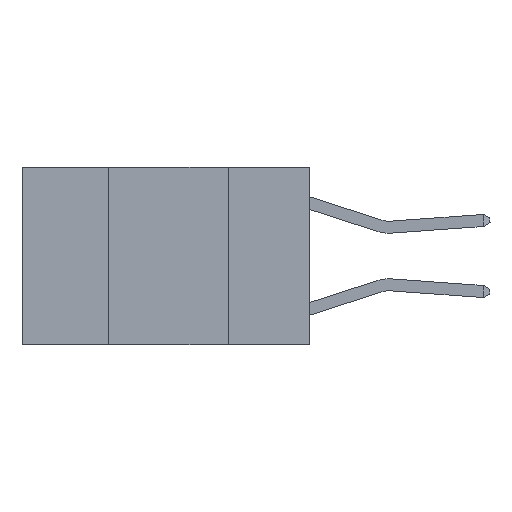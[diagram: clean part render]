
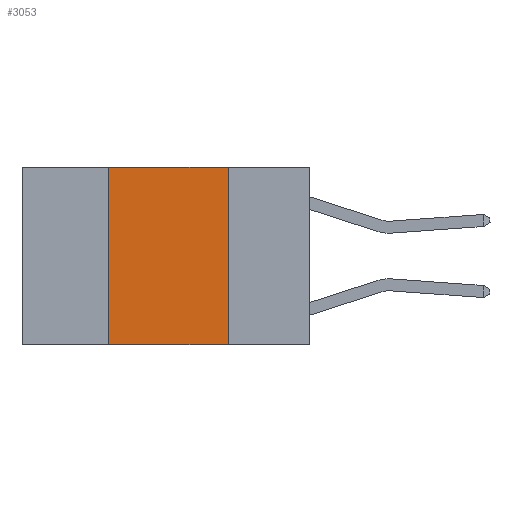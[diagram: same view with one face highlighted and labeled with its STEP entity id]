
A CAD part, left-side view. The second image highlights one B-rep face of the part: STEP entity #3053.
In plain terms, the highlighted planar face has unit normal (-1, 0, 0).
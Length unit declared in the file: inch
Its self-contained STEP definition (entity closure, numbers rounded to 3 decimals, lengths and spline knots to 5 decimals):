
#655 = VECTOR ( 'NONE', #10070, 39.37008 ) ;
#733 = PLANE ( 'NONE',  #889 ) ;
#889 = AXIS2_PLACEMENT_3D ( 'NONE', #7537, #8256, #3451 ) ;
#1529 = LINE ( 'NONE', #8002, #655 ) ;
#1813 = EDGE_CURVE ( 'NONE', #2491, #2219, #2151, .T. ) ;
#1826 = EDGE_LOOP ( 'NONE', ( #6441, #3651, #5259, #5713 ) ) ;
#2132 = CARTESIAN_POINT ( 'NONE',  ( 0., 0.6, 0. ) ) ;
#2151 = LINE ( 'NONE', #4082, #3375 ) ;
#2219 = VERTEX_POINT ( 'NONE', #6234 ) ;
#2269 = DIRECTION ( 'NONE',  ( 0., 0., -1. ) ) ;
#2373 = EDGE_CURVE ( 'NONE', #7387, #6988, #5102, .T. ) ;
#2491 = VERTEX_POINT ( 'NONE', #3180 ) ;
#3053 = ADVANCED_FACE ( 'NONE', ( #6031 ), #733, .F. ) ;
#3180 = CARTESIAN_POINT ( 'NONE',  ( 0., 0.42, -0.37 ) ) ;
#3375 = VECTOR ( 'NONE', #8993, 39.37008 ) ;
#3451 = DIRECTION ( 'NONE',  ( 0., 0., -1. ) ) ;
#3651 = ORIENTED_EDGE ( 'NONE', *, *, #2373, .F. ) ;
#4082 = CARTESIAN_POINT ( 'NONE',  ( 0., 0.6, -0.37 ) ) ;
#4575 = VECTOR ( 'NONE', #8576, 39.37008 ) ;
#5102 = LINE ( 'NONE', #2132, #4575 ) ;
#5259 = ORIENTED_EDGE ( 'NONE', *, *, #6414, .F. ) ;
#5412 = LINE ( 'NONE', #5809, #7459 ) ;
#5713 = ORIENTED_EDGE ( 'NONE', *, *, #1813, .T. ) ;
#5809 = CARTESIAN_POINT ( 'NONE',  ( 0., 0.17, 0. ) ) ;
#5831 = CARTESIAN_POINT ( 'NONE',  ( 0., 0.17, 0. ) ) ;
#6031 = FACE_OUTER_BOUND ( 'NONE', #1826, .T. ) ;
#6234 = CARTESIAN_POINT ( 'NONE',  ( 0., 0.17, -0.37 ) ) ;
#6414 = EDGE_CURVE ( 'NONE', #2491, #7387, #1529, .T. ) ;
#6418 = EDGE_CURVE ( 'NONE', #6988, #2219, #5412, .T. ) ;
#6441 = ORIENTED_EDGE ( 'NONE', *, *, #6418, .F. ) ;
#6988 = VERTEX_POINT ( 'NONE', #5831 ) ;
#7387 = VERTEX_POINT ( 'NONE', #8239 ) ;
#7459 = VECTOR ( 'NONE', #2269, 39.37008 ) ;
#7537 = CARTESIAN_POINT ( 'NONE',  ( 0., 0.6, 0. ) ) ;
#8002 = CARTESIAN_POINT ( 'NONE',  ( 0., 0.42, 0. ) ) ;
#8239 = CARTESIAN_POINT ( 'NONE',  ( 0., 0.42, 0. ) ) ;
#8256 = DIRECTION ( 'NONE',  ( 1., 0., 0. ) ) ;
#8576 = DIRECTION ( 'NONE',  ( 0., -1., 0. ) ) ;
#8993 = DIRECTION ( 'NONE',  ( 0., -1., 0. ) ) ;
#10070 = DIRECTION ( 'NONE',  ( 0., 0., 1. ) ) ;
